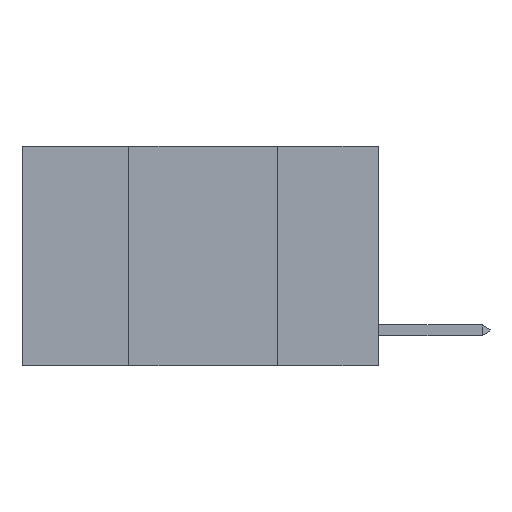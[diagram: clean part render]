
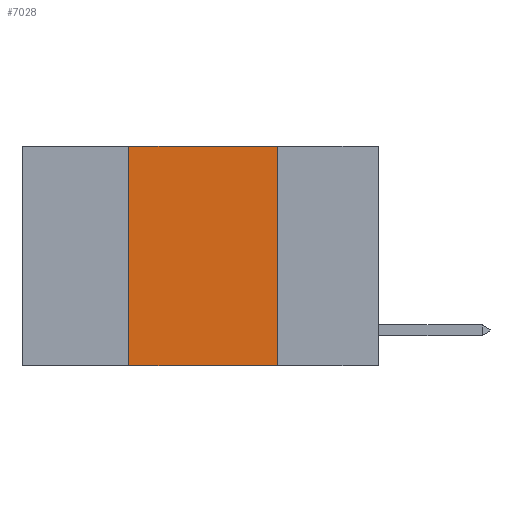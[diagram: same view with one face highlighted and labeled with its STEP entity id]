
A CAD part, left-side view. The second image highlights one B-rep face of the part: STEP entity #7028.
In plain terms, the highlighted planar face has unit normal (-1, 0, 0).
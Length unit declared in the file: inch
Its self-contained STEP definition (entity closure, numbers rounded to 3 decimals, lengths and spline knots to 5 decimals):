
#519 = CARTESIAN_POINT ( 'NONE',  ( 0., 0.42, -0.37 ) ) ;
#658 = EDGE_CURVE ( 'NONE', #2187, #2068, #6882, .T. ) ;
#1046 = CARTESIAN_POINT ( 'NONE',  ( 0., 0.42, 0. ) ) ;
#1373 = EDGE_CURVE ( 'NONE', #2392, #10160, #6587, .T. ) ;
#1399 = CARTESIAN_POINT ( 'NONE',  ( 0., 0.6, 0. ) ) ;
#1497 = AXIS2_PLACEMENT_3D ( 'NONE', #4012, #9899, #4931 ) ;
#1843 = DIRECTION ( 'NONE',  ( 0., 0., -1. ) ) ;
#2068 = VERTEX_POINT ( 'NONE', #5938 ) ;
#2187 = VERTEX_POINT ( 'NONE', #519 ) ;
#2392 = VERTEX_POINT ( 'NONE', #1046 ) ;
#2409 = DIRECTION ( 'NONE',  ( 0., -1., 0. ) ) ;
#2706 = ORIENTED_EDGE ( 'NONE', *, *, #4676, .F. ) ;
#2826 = EDGE_CURVE ( 'NONE', #2187, #2392, #6348, .T. ) ;
#3002 = CARTESIAN_POINT ( 'NONE',  ( 0., 0.6, -0.37 ) ) ;
#3025 = ORIENTED_EDGE ( 'NONE', *, *, #2826, .F. ) ;
#4012 = CARTESIAN_POINT ( 'NONE',  ( 0., 0.6, 0. ) ) ;
#4676 = EDGE_CURVE ( 'NONE', #10160, #2068, #4890, .T. ) ;
#4830 = CARTESIAN_POINT ( 'NONE',  ( 0., 0.17, 0. ) ) ;
#4890 = LINE ( 'NONE', #4830, #9057 ) ;
#4931 = DIRECTION ( 'NONE',  ( 0., 0., -1. ) ) ;
#5267 = ORIENTED_EDGE ( 'NONE', *, *, #1373, .F. ) ;
#5527 = ORIENTED_EDGE ( 'NONE', *, *, #658, .T. ) ;
#5938 = CARTESIAN_POINT ( 'NONE',  ( 0., 0.17, -0.37 ) ) ;
#5964 = DIRECTION ( 'NONE',  ( 0., -1., 0. ) ) ;
#6085 = VECTOR ( 'NONE', #8423, 39.37008 ) ;
#6348 = LINE ( 'NONE', #7566, #6085 ) ;
#6587 = LINE ( 'NONE', #1399, #10745 ) ;
#6594 = CARTESIAN_POINT ( 'NONE',  ( 0., 0.17, 0. ) ) ;
#6882 = LINE ( 'NONE', #3002, #11257 ) ;
#7028 = ADVANCED_FACE ( 'NONE', ( #9157 ), #11440, .F. ) ;
#7566 = CARTESIAN_POINT ( 'NONE',  ( 0., 0.42, 0. ) ) ;
#8423 = DIRECTION ( 'NONE',  ( 0., 0., 1. ) ) ;
#9057 = VECTOR ( 'NONE', #1843, 39.37008 ) ;
#9157 = FACE_OUTER_BOUND ( 'NONE', #11174, .T. ) ;
#9899 = DIRECTION ( 'NONE',  ( 1., 0., 0. ) ) ;
#10160 = VERTEX_POINT ( 'NONE', #6594 ) ;
#10745 = VECTOR ( 'NONE', #2409, 39.37008 ) ;
#11174 = EDGE_LOOP ( 'NONE', ( #2706, #5267, #3025, #5527 ) ) ;
#11257 = VECTOR ( 'NONE', #5964, 39.37008 ) ;
#11440 = PLANE ( 'NONE',  #1497 ) ;
